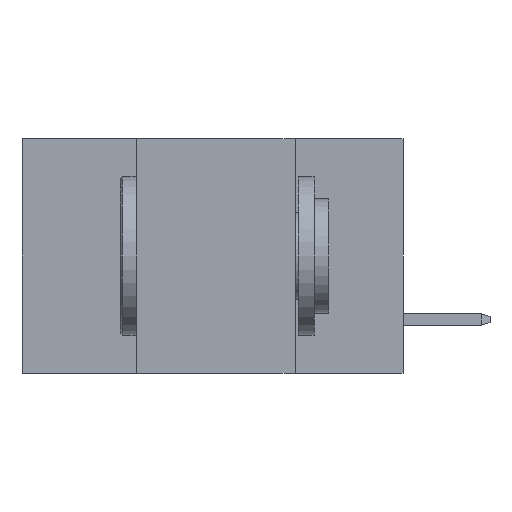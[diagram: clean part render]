
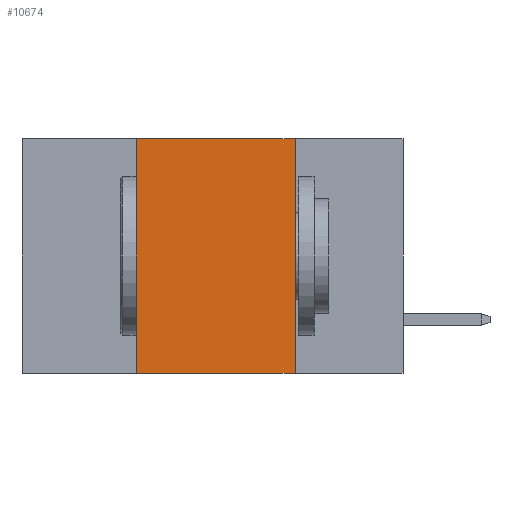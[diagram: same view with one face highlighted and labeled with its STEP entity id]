
A CAD part, left-side view. The second image highlights one B-rep face of the part: STEP entity #10674.
In plain terms, the highlighted planar face has unit normal (-1, 0, 0).
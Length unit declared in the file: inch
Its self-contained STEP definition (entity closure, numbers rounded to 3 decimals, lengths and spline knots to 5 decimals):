
#5 = VERTEX_POINT ( 'NONE', #4838 ) ;
#178 = EDGE_LOOP ( 'NONE', ( #5218, #6476, #4066, #4563 ) ) ;
#294 = VECTOR ( 'NONE', #4157, 39.37008 ) ;
#319 = CARTESIAN_POINT ( 'NONE',  ( 0., 0.6, 0. ) ) ;
#927 = VERTEX_POINT ( 'NONE', #2578 ) ;
#1241 = EDGE_CURVE ( 'NONE', #5, #10087, #11280, .T. ) ;
#1741 = VECTOR ( 'NONE', #4147, 39.37008 ) ;
#2011 = DIRECTION ( 'NONE',  ( 1., 0., 0. ) ) ;
#2407 = VECTOR ( 'NONE', #9746, 39.37008 ) ;
#2428 = CARTESIAN_POINT ( 'NONE',  ( 0., 0.42, 0. ) ) ;
#2545 = EDGE_CURVE ( 'NONE', #5, #6176, #6852, .T. ) ;
#2578 = CARTESIAN_POINT ( 'NONE',  ( 0., 0.17, 0. ) ) ;
#3467 = EDGE_CURVE ( 'NONE', #6176, #927, #5956, .T. ) ;
#3652 = CARTESIAN_POINT ( 'NONE',  ( 0., 0.42, 0. ) ) ;
#3877 = DIRECTION ( 'NONE',  ( 0., 0., -1. ) ) ;
#4066 = ORIENTED_EDGE ( 'NONE', *, *, #2545, .F. ) ;
#4147 = DIRECTION ( 'NONE',  ( 0., -1., 0. ) ) ;
#4157 = DIRECTION ( 'NONE',  ( 0., -1., 0. ) ) ;
#4260 = CARTESIAN_POINT ( 'NONE',  ( 0., 0.6, -0.37 ) ) ;
#4563 = ORIENTED_EDGE ( 'NONE', *, *, #1241, .T. ) ;
#4758 = FACE_OUTER_BOUND ( 'NONE', #178, .T. ) ;
#4838 = CARTESIAN_POINT ( 'NONE',  ( 0., 0.42, -0.37 ) ) ;
#5218 = ORIENTED_EDGE ( 'NONE', *, *, #10540, .F. ) ;
#5956 = LINE ( 'NONE', #6774, #294 ) ;
#5990 = DIRECTION ( 'NONE',  ( 0., 0., 1. ) ) ;
#6176 = VERTEX_POINT ( 'NONE', #3652 ) ;
#6213 = LINE ( 'NONE', #7893, #2407 ) ;
#6476 = ORIENTED_EDGE ( 'NONE', *, *, #3467, .F. ) ;
#6774 = CARTESIAN_POINT ( 'NONE',  ( 0., 0.6, 0. ) ) ;
#6852 = LINE ( 'NONE', #2428, #8470 ) ;
#7028 = CARTESIAN_POINT ( 'NONE',  ( 0., 0.17, -0.37 ) ) ;
#7893 = CARTESIAN_POINT ( 'NONE',  ( 0., 0.17, 0. ) ) ;
#8131 = PLANE ( 'NONE',  #10570 ) ;
#8470 = VECTOR ( 'NONE', #5990, 39.37008 ) ;
#9746 = DIRECTION ( 'NONE',  ( 0., 0., -1. ) ) ;
#10087 = VERTEX_POINT ( 'NONE', #7028 ) ;
#10540 = EDGE_CURVE ( 'NONE', #927, #10087, #6213, .T. ) ;
#10570 = AXIS2_PLACEMENT_3D ( 'NONE', #319, #2011, #3877 ) ;
#10674 = ADVANCED_FACE ( 'NONE', ( #4758 ), #8131, .F. ) ;
#11280 = LINE ( 'NONE', #4260, #1741 ) ;
